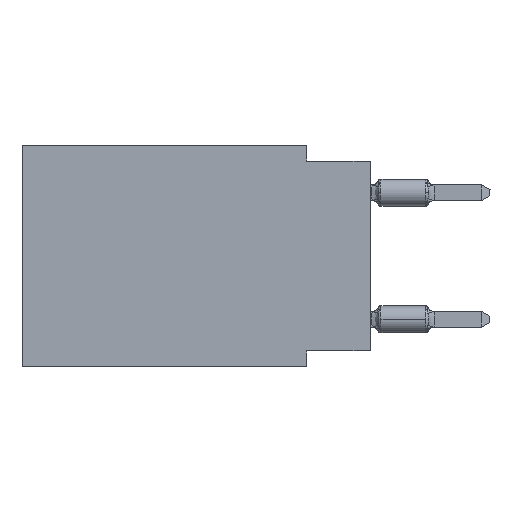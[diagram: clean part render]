
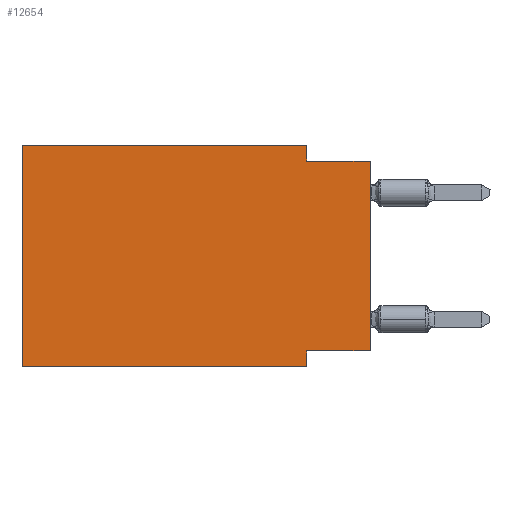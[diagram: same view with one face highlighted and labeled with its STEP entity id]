
A CAD part, left-side view. The second image highlights one B-rep face of the part: STEP entity #12654.
In plain terms, the highlighted planar face has unit normal (-1, 0, 0).
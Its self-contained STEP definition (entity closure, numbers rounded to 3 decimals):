
#560 = CARTESIAN_POINT ( 'NONE',  ( 0., 13.97, 0. ) ) ;
#1464 = VERTEX_POINT ( 'NONE', #11847 ) ;
#2299 = ORIENTED_EDGE ( 'NONE', *, *, #5781, .T. ) ;
#2628 = VERTEX_POINT ( 'NONE', #24310 ) ;
#2731 = LINE ( 'NONE', #23131, #22334 ) ;
#3274 = ORIENTED_EDGE ( 'NONE', *, *, #21187, .F. ) ;
#3863 = VERTEX_POINT ( 'NONE', #12295 ) ;
#4999 = DIRECTION ( 'NONE',  ( 0., 1., 0. ) ) ;
#5781 = EDGE_CURVE ( 'NONE', #2628, #25892, #15802, .T. ) ;
#5822 = ORIENTED_EDGE ( 'NONE', *, *, #21326, .F. ) ;
#6460 = ORIENTED_EDGE ( 'NONE', *, *, #8202, .F. ) ;
#6472 = VECTOR ( 'NONE', #23458, 1000. ) ;
#7885 = CARTESIAN_POINT ( 'NONE',  ( 0., 13.97, -8.89 ) ) ;
#8202 = EDGE_CURVE ( 'NONE', #9062, #1464, #18957, .T. ) ;
#8386 = FACE_OUTER_BOUND ( 'NONE', #14812, .T. ) ;
#8467 = VECTOR ( 'NONE', #12617, 1000. ) ;
#8707 = ORIENTED_EDGE ( 'NONE', *, *, #23752, .T. ) ;
#9062 = VERTEX_POINT ( 'NONE', #15765 ) ;
#9702 = ORIENTED_EDGE ( 'NONE', *, *, #25109, .F. ) ;
#10133 = CARTESIAN_POINT ( 'NONE',  ( 0., 13.97, 0. ) ) ;
#10176 = LINE ( 'NONE', #26546, #22593 ) ;
#10341 = EDGE_CURVE ( 'NONE', #1464, #24689, #25835, .T. ) ;
#11847 = CARTESIAN_POINT ( 'NONE',  ( 0., 2.54, 0. ) ) ;
#11937 = VECTOR ( 'NONE', #14513, 1000. ) ;
#12295 = CARTESIAN_POINT ( 'NONE',  ( 0., 0., -0.635 ) ) ;
#12617 = DIRECTION ( 'NONE',  ( 0., -1., 0. ) ) ;
#12654 = ADVANCED_FACE ( 'NONE', ( #8386 ), #24878, .F. ) ;
#12757 = VERTEX_POINT ( 'NONE', #17499 ) ;
#13008 = CARTESIAN_POINT ( 'NONE',  ( 0., 0., -0.635 ) ) ;
#13096 = CARTESIAN_POINT ( 'NONE',  ( 0., 2.54, -8.255 ) ) ;
#14346 = DIRECTION ( 'NONE',  ( 0., 0., 1. ) ) ;
#14479 = LINE ( 'NONE', #13008, #8467 ) ;
#14513 = DIRECTION ( 'NONE',  ( 0., 0., 1. ) ) ;
#14651 = CARTESIAN_POINT ( 'NONE',  ( 0., 2.54, -8.89 ) ) ;
#14667 = ORIENTED_EDGE ( 'NONE', *, *, #25776, .F. ) ;
#14678 = VECTOR ( 'NONE', #23103, 1000. ) ;
#14694 = DIRECTION ( 'NONE',  ( 1., 0., 0. ) ) ;
#14812 = EDGE_LOOP ( 'NONE', ( #8707, #9702, #20577, #6460, #14667, #2299, #3274, #5822 ) ) ;
#15645 = CARTESIAN_POINT ( 'NONE',  ( 0., 2.54, 0. ) ) ;
#15765 = CARTESIAN_POINT ( 'NONE',  ( 0., 13.97, 0. ) ) ;
#15802 = LINE ( 'NONE', #7885, #23667 ) ;
#16663 = CARTESIAN_POINT ( 'NONE',  ( 0., 2.54, -0.635 ) ) ;
#17499 = CARTESIAN_POINT ( 'NONE',  ( 0., 0., -8.255 ) ) ;
#18957 = LINE ( 'NONE', #560, #14678 ) ;
#19297 = CARTESIAN_POINT ( 'NONE',  ( 0., 2.54, -8.89 ) ) ;
#19988 = VERTEX_POINT ( 'NONE', #13096 ) ;
#20197 = AXIS2_PLACEMENT_3D ( 'NONE', #10133, #14694, #24748 ) ;
#20296 = CARTESIAN_POINT ( 'NONE',  ( 0., 13.97, 0. ) ) ;
#20372 = DIRECTION ( 'NONE',  ( 0., -1., 0. ) ) ;
#20577 = ORIENTED_EDGE ( 'NONE', *, *, #10341, .F. ) ;
#21187 = EDGE_CURVE ( 'NONE', #19988, #25892, #23336, .T. ) ;
#21326 = EDGE_CURVE ( 'NONE', #12757, #19988, #2731, .T. ) ;
#22334 = VECTOR ( 'NONE', #4999, 1000. ) ;
#22593 = VECTOR ( 'NONE', #14346, 1000. ) ;
#23103 = DIRECTION ( 'NONE',  ( 0., -1., 0. ) ) ;
#23131 = CARTESIAN_POINT ( 'NONE',  ( 0., 0., -8.255 ) ) ;
#23336 = LINE ( 'NONE', #19297, #6472 ) ;
#23458 = DIRECTION ( 'NONE',  ( 0., 0., -1. ) ) ;
#23667 = VECTOR ( 'NONE', #20372, 1000. ) ;
#23752 = EDGE_CURVE ( 'NONE', #12757, #3863, #10176, .T. ) ;
#23820 = DIRECTION ( 'NONE',  ( 0., 0., -1. ) ) ;
#24136 = VECTOR ( 'NONE', #23820, 1000. ) ;
#24310 = CARTESIAN_POINT ( 'NONE',  ( 0., 13.97, -8.89 ) ) ;
#24689 = VERTEX_POINT ( 'NONE', #16663 ) ;
#24704 = LINE ( 'NONE', #20296, #11937 ) ;
#24748 = DIRECTION ( 'NONE',  ( 0., 0., -1. ) ) ;
#24878 = PLANE ( 'NONE',  #20197 ) ;
#25109 = EDGE_CURVE ( 'NONE', #24689, #3863, #14479, .T. ) ;
#25776 = EDGE_CURVE ( 'NONE', #2628, #9062, #24704, .T. ) ;
#25835 = LINE ( 'NONE', #15645, #24136 ) ;
#25892 = VERTEX_POINT ( 'NONE', #14651 ) ;
#26546 = CARTESIAN_POINT ( 'NONE',  ( 0., 0., 0. ) ) ;
